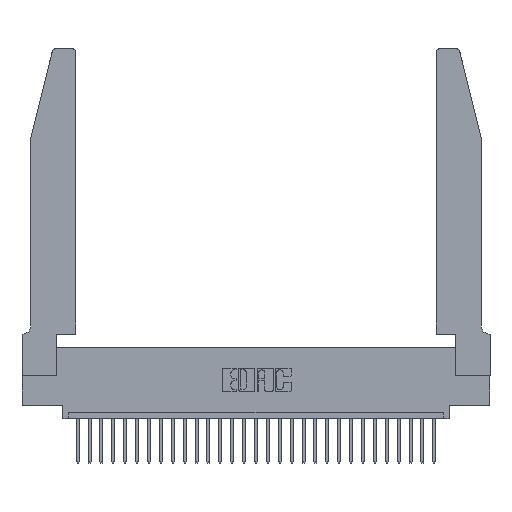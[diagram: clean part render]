
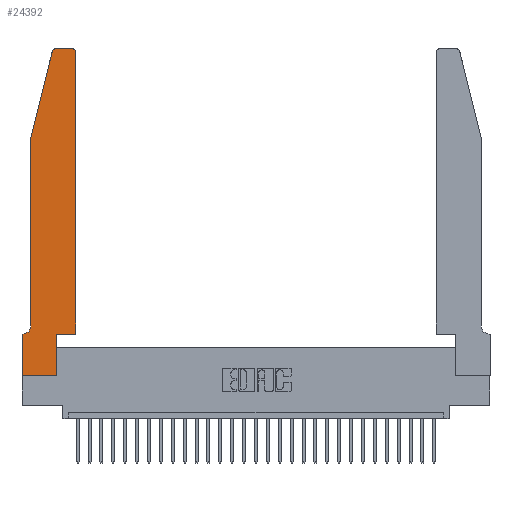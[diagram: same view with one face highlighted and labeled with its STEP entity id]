
A CAD part, top view. The second image highlights one B-rep face of the part: STEP entity #24392.
In plain terms, the highlighted planar face has unit normal (0, 0, 1).
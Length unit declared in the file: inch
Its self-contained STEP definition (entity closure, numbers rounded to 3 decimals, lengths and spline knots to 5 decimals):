
#306 = CARTESIAN_POINT ( 'NONE',  ( 0.0755, 0.35, 0.37 ) ) ;
#671 = LINE ( 'NONE', #8847, #20091 ) ;
#829 = CARTESIAN_POINT ( 'NONE',  ( 0.2865, 0.35, 0.37 ) ) ;
#988 = ORIENTED_EDGE ( 'NONE', *, *, #7547, .T. ) ;
#1189 = CARTESIAN_POINT ( 'NONE',  ( 0.284, 2.75, 0.37 ) ) ;
#1306 = ORIENTED_EDGE ( 'NONE', *, *, #23044, .T. ) ;
#1553 = EDGE_CURVE ( 'NONE', #2347, #13395, #2826, .T. ) ;
#1967 = AXIS2_PLACEMENT_3D ( 'NONE', #8043, #3369, #10156 ) ;
#2347 = VERTEX_POINT ( 'NONE', #27110 ) ;
#2477 = DIRECTION ( 'NONE',  ( 0., 1., 0. ) ) ;
#2612 = LINE ( 'NONE', #22770, #10874 ) ;
#2617 = DIRECTION ( 'NONE',  ( -1., 0., 0. ) ) ;
#2655 = ORIENTED_EDGE ( 'NONE', *, *, #16848, .T. ) ;
#2661 = CARTESIAN_POINT ( 'NONE',  ( 0., 0.35, 0.37 ) ) ;
#2826 = LINE ( 'NONE', #6990, #28675 ) ;
#3369 = DIRECTION ( 'NONE',  ( 0., 0., -1. ) ) ;
#3462 = ORIENTED_EDGE ( 'NONE', *, *, #1553, .T. ) ;
#3578 = VECTOR ( 'NONE', #17428, 39.37008 ) ;
#3676 = CARTESIAN_POINT ( 'NONE',  ( 0.4505, 2.72, 0.37 ) ) ;
#3785 = VECTOR ( 'NONE', #24224, 39.37008 ) ;
#4429 = ORIENTED_EDGE ( 'NONE', *, *, #23266, .T. ) ;
#4589 = PLANE ( 'NONE',  #24276 ) ;
#4862 = CIRCLE ( 'NONE', #24625, 0.03 ) ;
#5001 = CARTESIAN_POINT ( 'NONE',  ( 0.25487, 2.72718, 0.37 ) ) ;
#5174 = DIRECTION ( 'NONE',  ( 0., 0., 1. ) ) ;
#5255 = VERTEX_POINT ( 'NONE', #27827 ) ;
#5686 = CARTESIAN_POINT ( 'NONE',  ( 0.0055, 0.35, 0.37 ) ) ;
#5900 = CIRCLE ( 'NONE', #17375, 0.03 ) ;
#5992 = FACE_OUTER_BOUND ( 'NONE', #29297, .T. ) ;
#6110 = CARTESIAN_POINT ( 'NONE',  ( 0., 0., 0.37 ) ) ;
#6279 = VERTEX_POINT ( 'NONE', #21849 ) ;
#6851 = CARTESIAN_POINT ( 'NONE',  ( 0.284, 2.72, 0.37 ) ) ;
#6986 = ORIENTED_EDGE ( 'NONE', *, *, #14553, .T. ) ;
#6990 = CARTESIAN_POINT ( 'NONE',  ( 0.2865, 0.35, 0.37 ) ) ;
#7455 = DIRECTION ( 'NONE',  ( 1., 0., 0. ) ) ;
#7470 = LINE ( 'NONE', #16754, #24345 ) ;
#7547 = EDGE_CURVE ( 'NONE', #29156, #21181, #5900, .T. ) ;
#7580 = DIRECTION ( 'NONE',  ( 1., 0., 0. ) ) ;
#7638 = EDGE_CURVE ( 'NONE', #14004, #14747, #13063, .T. ) ;
#7681 = DIRECTION ( 'NONE',  ( -1., 0., 0. ) ) ;
#8043 = CARTESIAN_POINT ( 'NONE',  ( 0.0055, 0.42, 0.37 ) ) ;
#8847 = CARTESIAN_POINT ( 'NONE',  ( 0.0755, 2., 0.37 ) ) ;
#9639 = LINE ( 'NONE', #12888, #3578 ) ;
#10156 = DIRECTION ( 'NONE',  ( -1., 0., 0. ) ) ;
#10162 = VERTEX_POINT ( 'NONE', #3676 ) ;
#10874 = VECTOR ( 'NONE', #22478, 39.37008 ) ;
#11659 = DIRECTION ( 'NONE',  ( 0., 0., 1. ) ) ;
#12888 = CARTESIAN_POINT ( 'NONE',  ( 0.4505, 0.35, 0.37 ) ) ;
#13063 = LINE ( 'NONE', #306, #18095 ) ;
#13395 = VERTEX_POINT ( 'NONE', #829 ) ;
#14004 = VERTEX_POINT ( 'NONE', #5686 ) ;
#14403 = CARTESIAN_POINT ( 'NONE',  ( 0.0755, 0.42, 0.37 ) ) ;
#14553 = EDGE_CURVE ( 'NONE', #5255, #10162, #9639, .T. ) ;
#14747 = VERTEX_POINT ( 'NONE', #29449 ) ;
#15224 = VERTEX_POINT ( 'NONE', #14403 ) ;
#15856 = VECTOR ( 'NONE', #7681, 39.37008 ) ;
#16754 = CARTESIAN_POINT ( 'NONE',  ( 0.4505, 0.35, 0.37 ) ) ;
#16789 = CARTESIAN_POINT ( 'NONE',  ( 0.4205, 2.72, 0.37 ) ) ;
#16848 = EDGE_CURVE ( 'NONE', #28860, #15224, #29230, .T. ) ;
#17375 = AXIS2_PLACEMENT_3D ( 'NONE', #6851, #11659, #25298 ) ;
#17428 = DIRECTION ( 'NONE',  ( 0., 1., 0. ) ) ;
#17577 = VECTOR ( 'NONE', #19977, 39.37008 ) ;
#18095 = VECTOR ( 'NONE', #2617, 39.37008 ) ;
#19977 = DIRECTION ( 'NONE',  ( 1., 0., 0. ) ) ;
#20091 = VECTOR ( 'NONE', #29419, 39.37008 ) ;
#20674 = ORIENTED_EDGE ( 'NONE', *, *, #29582, .T. ) ;
#21138 = CIRCLE ( 'NONE', #1967, 0.07 ) ;
#21181 = VERTEX_POINT ( 'NONE', #5001 ) ;
#21200 = LINE ( 'NONE', #6110, #17577 ) ;
#21621 = ORIENTED_EDGE ( 'NONE', *, *, #26188, .T. ) ;
#21849 = CARTESIAN_POINT ( 'NONE',  ( 0.4205, 2.75, 0.37 ) ) ;
#22030 = CARTESIAN_POINT ( 'NONE',  ( 0.0755, 2., 0.37 ) ) ;
#22478 = DIRECTION ( 'NONE',  ( 0., -1., 0. ) ) ;
#22660 = CARTESIAN_POINT ( 'NONE',  ( 0., 0., 0.37 ) ) ;
#22770 = CARTESIAN_POINT ( 'NONE',  ( 0., 0., 0.37 ) ) ;
#22903 = EDGE_CURVE ( 'NONE', #15224, #14004, #21138, .T. ) ;
#23002 = ORIENTED_EDGE ( 'NONE', *, *, #23303, .T. ) ;
#23044 = EDGE_CURVE ( 'NONE', #21181, #28860, #671, .T. ) ;
#23266 = EDGE_CURVE ( 'NONE', #10162, #6279, #4862, .T. ) ;
#23303 = EDGE_CURVE ( 'NONE', #6279, #29156, #27366, .T. ) ;
#23750 = DIRECTION ( 'NONE',  ( 0., 0., 1. ) ) ;
#24224 = DIRECTION ( 'NONE',  ( 0., -1., 0. ) ) ;
#24276 = AXIS2_PLACEMENT_3D ( 'NONE', #2661, #5174, #7455 ) ;
#24345 = VECTOR ( 'NONE', #28544, 39.37008 ) ;
#24392 = ADVANCED_FACE ( 'NONE', ( #5992 ), #4589, .T. ) ;
#24625 = AXIS2_PLACEMENT_3D ( 'NONE', #16789, #23750, #7580 ) ;
#24689 = VERTEX_POINT ( 'NONE', #22660 ) ;
#25280 = ORIENTED_EDGE ( 'NONE', *, *, #22903, .T. ) ;
#25298 = DIRECTION ( 'NONE',  ( 1., 0., 0. ) ) ;
#25444 = CARTESIAN_POINT ( 'NONE',  ( 0.0755, 2., 0.37 ) ) ;
#26188 = EDGE_CURVE ( 'NONE', #14747, #24689, #2612, .T. ) ;
#26471 = ORIENTED_EDGE ( 'NONE', *, *, #28662, .T. ) ;
#27110 = CARTESIAN_POINT ( 'NONE',  ( 0.2865, 0., 0.37 ) ) ;
#27366 = LINE ( 'NONE', #28578, #15856 ) ;
#27827 = CARTESIAN_POINT ( 'NONE',  ( 0.4505, 0.35, 0.37 ) ) ;
#28544 = DIRECTION ( 'NONE',  ( 1., 0., 0. ) ) ;
#28578 = CARTESIAN_POINT ( 'NONE',  ( 0.2605, 2.75, 0.37 ) ) ;
#28662 = EDGE_CURVE ( 'NONE', #24689, #2347, #21200, .T. ) ;
#28675 = VECTOR ( 'NONE', #2477, 39.37008 ) ;
#28695 = ORIENTED_EDGE ( 'NONE', *, *, #7638, .T. ) ;
#28860 = VERTEX_POINT ( 'NONE', #25444 ) ;
#29156 = VERTEX_POINT ( 'NONE', #1189 ) ;
#29230 = LINE ( 'NONE', #22030, #3785 ) ;
#29297 = EDGE_LOOP ( 'NONE', ( #23002, #988, #1306, #2655, #25280, #28695, #21621, #26471, #3462, #20674, #6986, #4429 ) ) ;
#29419 = DIRECTION ( 'NONE',  ( -0.239, -0.971, 0. ) ) ;
#29449 = CARTESIAN_POINT ( 'NONE',  ( 0., 0.35, 0.37 ) ) ;
#29582 = EDGE_CURVE ( 'NONE', #13395, #5255, #7470, .T. ) ;
